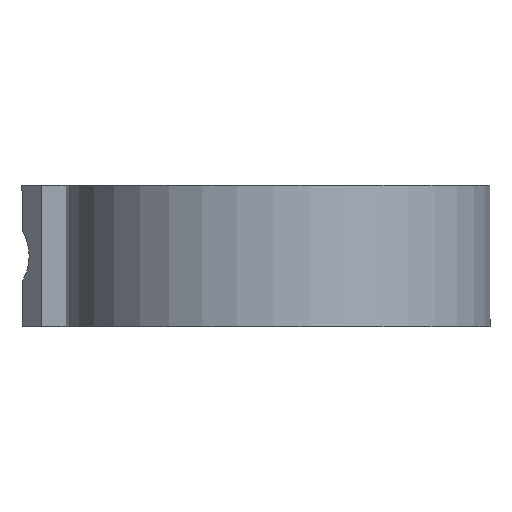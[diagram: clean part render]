
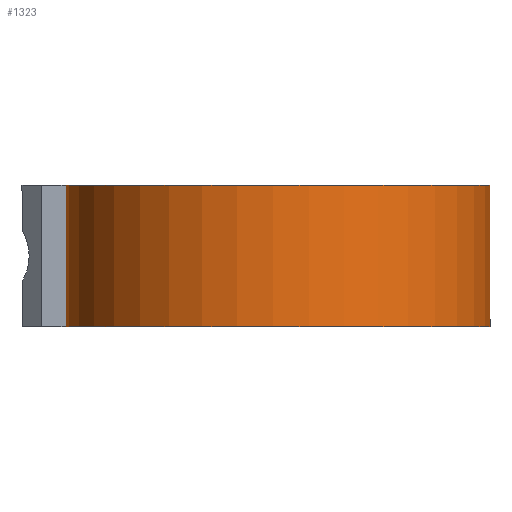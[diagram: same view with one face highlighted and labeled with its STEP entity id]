
A CAD part, front view. The second image highlights one B-rep face of the part: STEP entity #1323.
In plain terms, the highlighted cylindrical face has radius 15.24 mm (diameter 30.48 mm), a partial arc.
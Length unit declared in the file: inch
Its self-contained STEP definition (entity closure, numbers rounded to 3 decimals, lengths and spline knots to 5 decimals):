
#67 = VERTEX_POINT ( 'NONE', #1396 ) ;
#121 = VERTEX_POINT ( 'NONE', #1404 ) ;
#176 = DIRECTION ( 'NONE',  ( -1., 0., 0. ) ) ;
#186 = EDGE_CURVE ( 'NONE', #1094, #67, #937, .T. ) ;
#241 = ORIENTED_EDGE ( 'NONE', *, *, #186, .T. ) ;
#249 = AXIS2_PLACEMENT_3D ( 'NONE', #986, #489, #1075 ) ;
#254 = CARTESIAN_POINT ( 'NONE',  ( 0.7775, 0.04871, 0.90238 ) ) ;
#297 = VECTOR ( 'NONE', #511, 39.37008 ) ;
#313 = LINE ( 'NONE', #1457, #297 ) ;
#395 = DIRECTION ( 'NONE',  ( 0., 0., -1. ) ) ;
#421 = EDGE_CURVE ( 'NONE', #121, #831, #313, .T. ) ;
#443 = ORIENTED_EDGE ( 'NONE', *, *, #421, .T. ) ;
#489 = DIRECTION ( 'NONE',  ( 0., 0., -1. ) ) ;
#511 = DIRECTION ( 'NONE',  ( 0., 0., -1. ) ) ;
#566 = DIRECTION ( 'NONE',  ( 1., 0., 0. ) ) ;
#601 = CARTESIAN_POINT ( 'NONE',  ( 0.3625, -0.38462, -1.14042 ) ) ;
#653 = EDGE_CURVE ( 'NONE', #831, #1094, #1468, .T. ) ;
#734 = AXIS2_PLACEMENT_3D ( 'NONE', #1403, #1498, #566 ) ;
#831 = VERTEX_POINT ( 'NONE', #1195 ) ;
#834 = AXIS2_PLACEMENT_3D ( 'NONE', #601, #395, #176 ) ;
#859 = VECTOR ( 'NONE', #1067, 39.37008 ) ;
#937 = LINE ( 'NONE', #254, #859 ) ;
#962 = EDGE_CURVE ( 'NONE', #67, #121, #991, .T. ) ;
#986 = CARTESIAN_POINT ( 'NONE',  ( 0.3625, -0.38462, 0.90238 ) ) ;
#991 = CIRCLE ( 'NONE', #834, 0.6 ) ;
#1008 = CYLINDRICAL_SURFACE ( 'NONE', #249, 0.6 ) ;
#1067 = DIRECTION ( 'NONE',  ( 0., 0., 1. ) ) ;
#1074 = ORIENTED_EDGE ( 'NONE', *, *, #653, .T. ) ;
#1075 = DIRECTION ( 'NONE',  ( -1., 0., 0. ) ) ;
#1094 = VERTEX_POINT ( 'NONE', #1341 ) ;
#1151 = EDGE_LOOP ( 'NONE', ( #1257, #443, #1074, #241 ) ) ;
#1195 = CARTESIAN_POINT ( 'NONE',  ( -0.2375, -0.38462, -1.54042 ) ) ;
#1257 = ORIENTED_EDGE ( 'NONE', *, *, #962, .T. ) ;
#1322 = FACE_OUTER_BOUND ( 'NONE', #1151, .T. ) ;
#1323 = ADVANCED_FACE ( 'NONE', ( #1322 ), #1008, .T. ) ;
#1341 = CARTESIAN_POINT ( 'NONE',  ( 0.7775, 0.04871, -1.54042 ) ) ;
#1396 = CARTESIAN_POINT ( 'NONE',  ( 0.7775, 0.04871, -1.14042 ) ) ;
#1403 = CARTESIAN_POINT ( 'NONE',  ( 0.3625, -0.38462, -1.54042 ) ) ;
#1404 = CARTESIAN_POINT ( 'NONE',  ( -0.2375, -0.38462, -1.14042 ) ) ;
#1457 = CARTESIAN_POINT ( 'NONE',  ( -0.2375, -0.38462, 0.90238 ) ) ;
#1468 = CIRCLE ( 'NONE', #734, 0.6 ) ;
#1498 = DIRECTION ( 'NONE',  ( 0., 0., 1. ) ) ;
